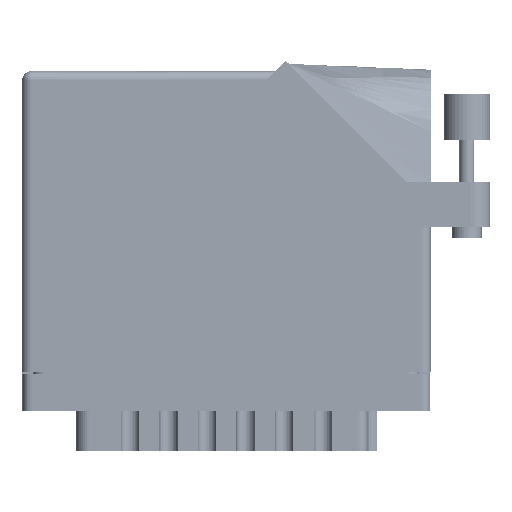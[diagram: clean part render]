
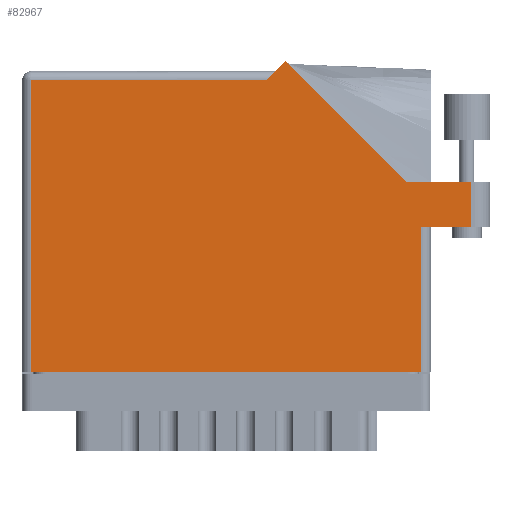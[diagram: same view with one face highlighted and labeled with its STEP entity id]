
A CAD part, front view. The second image highlights one B-rep face of the part: STEP entity #82967.
In plain terms, the highlighted face is planar.
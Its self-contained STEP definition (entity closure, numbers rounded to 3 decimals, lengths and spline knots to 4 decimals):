
#1448 = DIRECTION ( 'NONE',  ( 1., 0., 0. ) ) ;
#1706 = VERTEX_POINT ( 'NONE', #40885 ) ;
#2438 = VERTEX_POINT ( 'NONE', #81529 ) ;
#3401 = VECTOR ( 'NONE', #87016, 39.3701 ) ;
#5573 = CARTESIAN_POINT ( 'NONE',  ( 0.062, 0., 0. ) ) ;
#5587 = CARTESIAN_POINT ( 'NONE',  ( 3.03, 1.287, 0. ) ) ;
#8452 = VECTOR ( 'NONE', #1448, 39.3701 ) ;
#9556 = VECTOR ( 'NONE', #70065, 39.3701 ) ;
#10200 = CARTESIAN_POINT ( 'NONE',  ( 3.03, 0.98, 0. ) ) ;
#11700 = CARTESIAN_POINT ( 'NONE',  ( 1.643, 1.968, 0. ) ) ;
#12258 = EDGE_CURVE ( 'NONE', #2438, #92097, #69998, .T. ) ;
#16103 = EDGE_CURVE ( 'NONE', #1706, #81189, #38831, .T. ) ;
#16333 = CARTESIAN_POINT ( 'NONE',  ( 2.5894, 1.287, 0. ) ) ;
#16378 = FACE_OUTER_BOUND ( 'NONE', #60278, .T. ) ;
#19439 = VERTEX_POINT ( 'NONE', #11700 ) ;
#20068 = VERTEX_POINT ( 'NONE', #49712 ) ;
#20504 = ORIENTED_EDGE ( 'NONE', *, *, #33697, .T. ) ;
#22318 = ORIENTED_EDGE ( 'NONE', *, *, #49533, .T. ) ;
#27035 = CARTESIAN_POINT ( 'NONE',  ( 3.155, 1.287, 0. ) ) ;
#28191 = VECTOR ( 'NONE', #54175, 39.3701 ) ;
#30377 = LINE ( 'NONE', #27035, #89901 ) ;
#30957 = CARTESIAN_POINT ( 'NONE',  ( 2.5894, 1.287, 0. ) ) ;
#31903 = DIRECTION ( 'NONE',  ( 1., 0., 0. ) ) ;
#33697 = EDGE_CURVE ( 'NONE', #46981, #36359, #30377, .T. ) ;
#34237 = AXIS2_PLACEMENT_3D ( 'NONE', #52071, #75841, #61186 ) ;
#34829 = LINE ( 'NONE', #87163, #92021 ) ;
#36359 = VERTEX_POINT ( 'NONE', #30957 ) ;
#38831 = LINE ( 'NONE', #44777, #8452 ) ;
#40885 = CARTESIAN_POINT ( 'NONE',  ( 2.693, 0.98, 0. ) ) ;
#41251 = ORIENTED_EDGE ( 'NONE', *, *, #12258, .T. ) ;
#41768 = EDGE_CURVE ( 'NONE', #36359, #79540, #85306, .T. ) ;
#42964 = CARTESIAN_POINT ( 'NONE',  ( 0.062, 0., 0. ) ) ;
#43910 = PLANE ( 'NONE',  #34237 ) ;
#44777 = CARTESIAN_POINT ( 'NONE',  ( 2.755, 0.98, 0. ) ) ;
#45766 = ORIENTED_EDGE ( 'NONE', *, *, #76305, .T. ) ;
#46139 = LINE ( 'NONE', #60384, #58871 ) ;
#46981 = VERTEX_POINT ( 'NONE', #52628 ) ;
#49533 = EDGE_CURVE ( 'NONE', #92097, #20068, #74508, .T. ) ;
#49712 = CARTESIAN_POINT ( 'NONE',  ( 2.693, 0., 0. ) ) ;
#49754 = VECTOR ( 'NONE', #49926, 39.3701 ) ;
#49926 = DIRECTION ( 'NONE',  ( 0., 1., 0. ) ) ;
#51938 = DIRECTION ( 'NONE',  ( -0.707, -0.707, 0. ) ) ;
#52071 = CARTESIAN_POINT ( 'NONE',  ( 0., 2.03, 0. ) ) ;
#52628 = CARTESIAN_POINT ( 'NONE',  ( 3.03, 1.287, 0. ) ) ;
#54175 = DIRECTION ( 'NONE',  ( -0.707, 0.707, 0. ) ) ;
#57590 = EDGE_CURVE ( 'NONE', #81189, #46981, #67267, .T. ) ;
#58871 = VECTOR ( 'NONE', #51938, 39.3701 ) ;
#60278 = EDGE_LOOP ( 'NONE', ( #68057, #62533, #20504, #93598, #45766, #94362, #41251, #22318, #84809 ) ) ;
#60384 = CARTESIAN_POINT ( 'NONE',  ( 1.705, 2.03, 0. ) ) ;
#61186 = DIRECTION ( 'NONE',  ( -1., 0., 0. ) ) ;
#62533 = ORIENTED_EDGE ( 'NONE', *, *, #57590, .T. ) ;
#62575 = CARTESIAN_POINT ( 'NONE',  ( 2.693, 0.98, 0. ) ) ;
#62666 = CARTESIAN_POINT ( 'NONE',  ( 1.7757, 2.1007, 0. ) ) ;
#65633 = LINE ( 'NONE', #62575, #9556 ) ;
#67267 = LINE ( 'NONE', #5587, #49754 ) ;
#67314 = DIRECTION ( 'NONE',  ( -1., 0., 0. ) ) ;
#68057 = ORIENTED_EDGE ( 'NONE', *, *, #16103, .T. ) ;
#68480 = CARTESIAN_POINT ( 'NONE',  ( 0., 0., 0. ) ) ;
#69998 = LINE ( 'NONE', #5573, #3401 ) ;
#70065 = DIRECTION ( 'NONE',  ( 0., 1., 0. ) ) ;
#74508 = LINE ( 'NONE', #68480, #80501 ) ;
#75841 = DIRECTION ( 'NONE',  ( 0., 0., -1. ) ) ;
#76305 = EDGE_CURVE ( 'NONE', #79540, #19439, #46139, .T. ) ;
#79201 = DIRECTION ( 'NONE',  ( -1., 0., 0. ) ) ;
#79540 = VERTEX_POINT ( 'NONE', #62666 ) ;
#80501 = VECTOR ( 'NONE', #31903, 39.3701 ) ;
#81189 = VERTEX_POINT ( 'NONE', #10200 ) ;
#81529 = CARTESIAN_POINT ( 'NONE',  ( 0.062, 1.968, 0. ) ) ;
#82967 = ADVANCED_FACE ( 'NONE', ( #16378 ), #43910, .F. ) ;
#84809 = ORIENTED_EDGE ( 'NONE', *, *, #86112, .T. ) ;
#85306 = LINE ( 'NONE', #16333, #28191 ) ;
#86112 = EDGE_CURVE ( 'NONE', #20068, #1706, #65633, .T. ) ;
#87016 = DIRECTION ( 'NONE',  ( 0., -1., 0. ) ) ;
#87163 = CARTESIAN_POINT ( 'NONE',  ( 0., 1.968, 0. ) ) ;
#89257 = EDGE_CURVE ( 'NONE', #19439, #2438, #34829, .T. ) ;
#89901 = VECTOR ( 'NONE', #79201, 39.3701 ) ;
#92021 = VECTOR ( 'NONE', #67314, 39.3701 ) ;
#92097 = VERTEX_POINT ( 'NONE', #42964 ) ;
#93598 = ORIENTED_EDGE ( 'NONE', *, *, #41768, .T. ) ;
#94362 = ORIENTED_EDGE ( 'NONE', *, *, #89257, .T. ) ;
